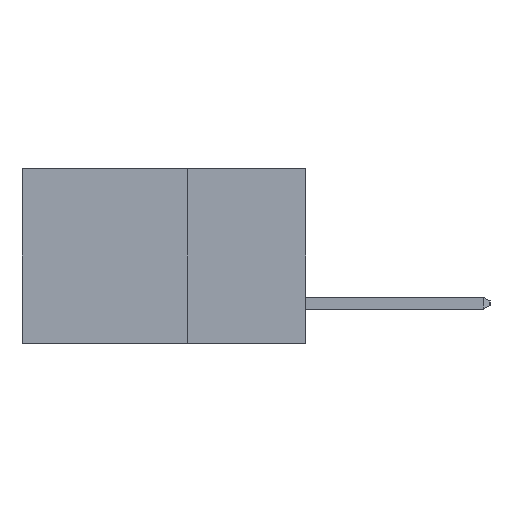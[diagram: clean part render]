
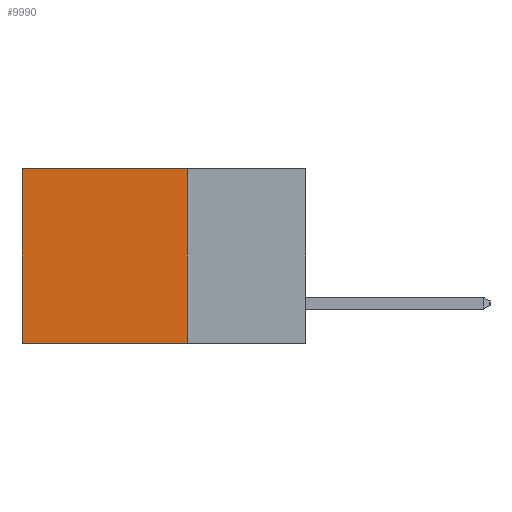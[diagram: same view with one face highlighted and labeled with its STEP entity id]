
A CAD part, left-side view. The second image highlights one B-rep face of the part: STEP entity #9990.
In plain terms, the highlighted planar face has unit normal (-1, 0, 0).
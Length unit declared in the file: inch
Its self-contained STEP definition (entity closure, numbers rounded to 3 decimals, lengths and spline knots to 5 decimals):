
#275 = ORIENTED_EDGE ( 'NONE', *, *, #6104, .F. ) ;
#371 = EDGE_LOOP ( 'NONE', ( #8966, #275, #9916, #9431 ) ) ;
#1330 = VECTOR ( 'NONE', #1719, 39.37008 ) ;
#1647 = DIRECTION ( 'NONE',  ( 0., 0., -1. ) ) ;
#1719 = DIRECTION ( 'NONE',  ( 0., 0., -1. ) ) ;
#2191 = LINE ( 'NONE', #9792, #10916 ) ;
#2210 = VERTEX_POINT ( 'NONE', #8889 ) ;
#2526 = EDGE_CURVE ( 'NONE', #2210, #10669, #3289, .T. ) ;
#2677 = CARTESIAN_POINT ( 'NONE',  ( 0.298, 0.25, 0. ) ) ;
#2969 = DIRECTION ( 'NONE',  ( 0., 1., 0. ) ) ;
#3098 = LINE ( 'NONE', #3893, #7330 ) ;
#3289 = LINE ( 'NONE', #8031, #1330 ) ;
#3893 = CARTESIAN_POINT ( 'NONE',  ( 0.298, 0.25, -0.37 ) ) ;
#5805 = VERTEX_POINT ( 'NONE', #2677 ) ;
#6104 = EDGE_CURVE ( 'NONE', #7700, #10669, #3098, .T. ) ;
#6469 = LINE ( 'NONE', #8918, #6739 ) ;
#6519 = AXIS2_PLACEMENT_3D ( 'NONE', #8385, #6664, #1647 ) ;
#6664 = DIRECTION ( 'NONE',  ( 1., 0., 0. ) ) ;
#6739 = VECTOR ( 'NONE', #2969, 39.37008 ) ;
#7280 = DIRECTION ( 'NONE',  ( 0., 1., 0. ) ) ;
#7330 = VECTOR ( 'NONE', #7280, 39.37008 ) ;
#7700 = VERTEX_POINT ( 'NONE', #7945 ) ;
#7945 = CARTESIAN_POINT ( 'NONE',  ( 0.298, 0.25, -0.37 ) ) ;
#8031 = CARTESIAN_POINT ( 'NONE',  ( 0.298, 0.6, 0. ) ) ;
#8385 = CARTESIAN_POINT ( 'NONE',  ( 0.298, 0.25, 0. ) ) ;
#8889 = CARTESIAN_POINT ( 'NONE',  ( 0.298, 0.6, 0. ) ) ;
#8918 = CARTESIAN_POINT ( 'NONE',  ( 0.298, 0.25, 0. ) ) ;
#8966 = ORIENTED_EDGE ( 'NONE', *, *, #2526, .T. ) ;
#9202 = CARTESIAN_POINT ( 'NONE',  ( 0.298, 0.6, -0.37 ) ) ;
#9431 = ORIENTED_EDGE ( 'NONE', *, *, #10392, .T. ) ;
#9776 = EDGE_CURVE ( 'NONE', #5805, #7700, #2191, .T. ) ;
#9792 = CARTESIAN_POINT ( 'NONE',  ( 0.298, 0.25, 0. ) ) ;
#9916 = ORIENTED_EDGE ( 'NONE', *, *, #9776, .F. ) ;
#9990 = ADVANCED_FACE ( 'NONE', ( #10526 ), #10072, .F. ) ;
#10072 = PLANE ( 'NONE',  #6519 ) ;
#10392 = EDGE_CURVE ( 'NONE', #5805, #2210, #6469, .T. ) ;
#10526 = FACE_OUTER_BOUND ( 'NONE', #371, .T. ) ;
#10648 = DIRECTION ( 'NONE',  ( 0., 0., -1. ) ) ;
#10669 = VERTEX_POINT ( 'NONE', #9202 ) ;
#10916 = VECTOR ( 'NONE', #10648, 39.37008 ) ;
